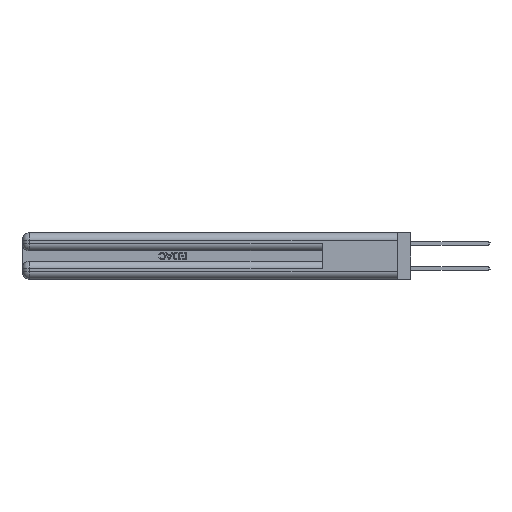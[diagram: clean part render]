
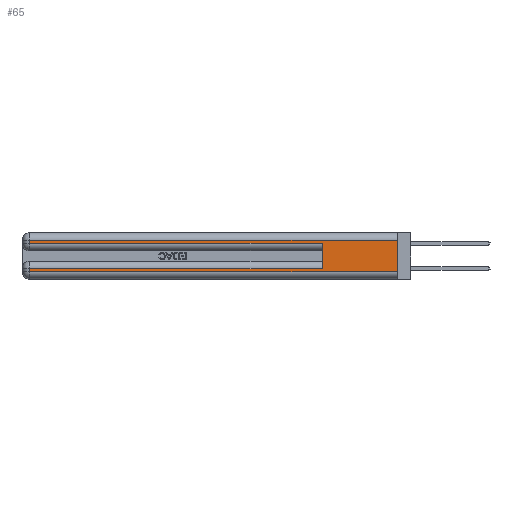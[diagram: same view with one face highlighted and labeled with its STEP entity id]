
A CAD part, left-side view. The second image highlights one B-rep face of the part: STEP entity #65.
In plain terms, the highlighted planar face has unit normal (-1, 0, 0).
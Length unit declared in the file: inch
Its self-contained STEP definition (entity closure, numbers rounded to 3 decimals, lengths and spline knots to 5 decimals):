
#65 = ADVANCED_FACE ( 'NONE', ( #50598 ), #15129, .F. ) ;
#734 = CARTESIAN_POINT ( 'NONE',  ( 0., 2.94, 0.37 ) ) ;
#1639 = CARTESIAN_POINT ( 'NONE',  ( 0., 2.94, 0.31 ) ) ;
#1768 = CARTESIAN_POINT ( 'NONE',  ( 0., 0., 0.085 ) ) ;
#2248 = EDGE_LOOP ( 'NONE', ( #47898, #25423, #30951, #34621, #38315, #15623, #49230, #19347 ) ) ;
#2334 = VERTEX_POINT ( 'NONE', #40286 ) ;
#3143 = CARTESIAN_POINT ( 'NONE',  ( 0., 0., 0.06 ) ) ;
#3411 = LINE ( 'NONE', #3143, #32320 ) ;
#4284 = LINE ( 'NONE', #1768, #44684 ) ;
#5439 = CARTESIAN_POINT ( 'NONE',  ( 0., 0., 0.31 ) ) ;
#5862 = CARTESIAN_POINT ( 'NONE',  ( 0., 2.94, 0.285 ) ) ;
#7901 = VECTOR ( 'NONE', #13536, 39.37008 ) ;
#9071 = LINE ( 'NONE', #41021, #49391 ) ;
#10177 = VECTOR ( 'NONE', #46284, 39.37008 ) ;
#12036 = EDGE_CURVE ( 'NONE', #14078, #18825, #49664, .T. ) ;
#12953 = DIRECTION ( 'NONE',  ( 0., 0., -1. ) ) ;
#13374 = DIRECTION ( 'NONE',  ( 0., 0., -1. ) ) ;
#13536 = DIRECTION ( 'NONE',  ( 0., 1., 0. ) ) ;
#14078 = VERTEX_POINT ( 'NONE', #5439 ) ;
#15050 = CARTESIAN_POINT ( 'NONE',  ( 0., 0.6, 0.145 ) ) ;
#15129 = PLANE ( 'NONE',  #33833 ) ;
#15623 = ORIENTED_EDGE ( 'NONE', *, *, #19582, .T. ) ;
#17328 = CARTESIAN_POINT ( 'NONE',  ( 0., 0., 0.06 ) ) ;
#18825 = VERTEX_POINT ( 'NONE', #17328 ) ;
#19089 = CARTESIAN_POINT ( 'NONE',  ( 0., 0., 0.37 ) ) ;
#19347 = ORIENTED_EDGE ( 'NONE', *, *, #45031, .T. ) ;
#19582 = EDGE_CURVE ( 'NONE', #24425, #2334, #4284, .T. ) ;
#19601 = LINE ( 'NONE', #44745, #7901 ) ;
#20607 = LINE ( 'NONE', #15050, #10177 ) ;
#21236 = EDGE_CURVE ( 'NONE', #32746, #43602, #9071, .T. ) ;
#21710 = CARTESIAN_POINT ( 'NONE',  ( 0., 0.6, 0.085 ) ) ;
#23019 = DIRECTION ( 'NONE',  ( 0., 0., -1. ) ) ;
#24425 = VERTEX_POINT ( 'NONE', #21710 ) ;
#24627 = CARTESIAN_POINT ( 'NONE',  ( 0., 2.94, 0.37 ) ) ;
#25423 = ORIENTED_EDGE ( 'NONE', *, *, #50590, .T. ) ;
#30492 = DIRECTION ( 'NONE',  ( 0., -1., 0. ) ) ;
#30951 = ORIENTED_EDGE ( 'NONE', *, *, #37656, .T. ) ;
#31065 = EDGE_CURVE ( 'NONE', #2334, #47342, #44811, .T. ) ;
#31451 = VECTOR ( 'NONE', #13374, 39.37008 ) ;
#32155 = LINE ( 'NONE', #24627, #41272 ) ;
#32200 = DIRECTION ( 'NONE',  ( 0., 0., -1. ) ) ;
#32320 = VECTOR ( 'NONE', #30492, 39.37008 ) ;
#32746 = VERTEX_POINT ( 'NONE', #5862 ) ;
#33412 = VERTEX_POINT ( 'NONE', #1639 ) ;
#33833 = AXIS2_PLACEMENT_3D ( 'NONE', #19089, #46352, #23019 ) ;
#34621 = ORIENTED_EDGE ( 'NONE', *, *, #21236, .T. ) ;
#37013 = CARTESIAN_POINT ( 'NONE',  ( 0., 0., 0.37 ) ) ;
#37656 = EDGE_CURVE ( 'NONE', #33412, #32746, #32155, .T. ) ;
#38315 = ORIENTED_EDGE ( 'NONE', *, *, #43098, .F. ) ;
#40286 = CARTESIAN_POINT ( 'NONE',  ( 0., 2.94, 0.085 ) ) ;
#41021 = CARTESIAN_POINT ( 'NONE',  ( 0., 0., 0.285 ) ) ;
#41272 = VECTOR ( 'NONE', #12953, 39.37008 ) ;
#42392 = VECTOR ( 'NONE', #32200, 39.37008 ) ;
#43098 = EDGE_CURVE ( 'NONE', #24425, #43602, #20607, .T. ) ;
#43602 = VERTEX_POINT ( 'NONE', #44345 ) ;
#44345 = CARTESIAN_POINT ( 'NONE',  ( 0., 0.6, 0.285 ) ) ;
#44684 = VECTOR ( 'NONE', #48830, 39.37008 ) ;
#44745 = CARTESIAN_POINT ( 'NONE',  ( 0., 0., 0.31 ) ) ;
#44811 = LINE ( 'NONE', #734, #42392 ) ;
#45031 = EDGE_CURVE ( 'NONE', #47342, #18825, #3411, .T. ) ;
#45326 = CARTESIAN_POINT ( 'NONE',  ( 0., 2.94, 0.06 ) ) ;
#46284 = DIRECTION ( 'NONE',  ( 0., 0., 1. ) ) ;
#46352 = DIRECTION ( 'NONE',  ( 1., 0., 0. ) ) ;
#47342 = VERTEX_POINT ( 'NONE', #45326 ) ;
#47898 = ORIENTED_EDGE ( 'NONE', *, *, #12036, .F. ) ;
#48819 = DIRECTION ( 'NONE',  ( 0., -1., 0. ) ) ;
#48830 = DIRECTION ( 'NONE',  ( 0., 1., 0. ) ) ;
#49230 = ORIENTED_EDGE ( 'NONE', *, *, #31065, .T. ) ;
#49391 = VECTOR ( 'NONE', #48819, 39.37008 ) ;
#49664 = LINE ( 'NONE', #37013, #31451 ) ;
#50590 = EDGE_CURVE ( 'NONE', #14078, #33412, #19601, .T. ) ;
#50598 = FACE_OUTER_BOUND ( 'NONE', #2248, .T. ) ;
